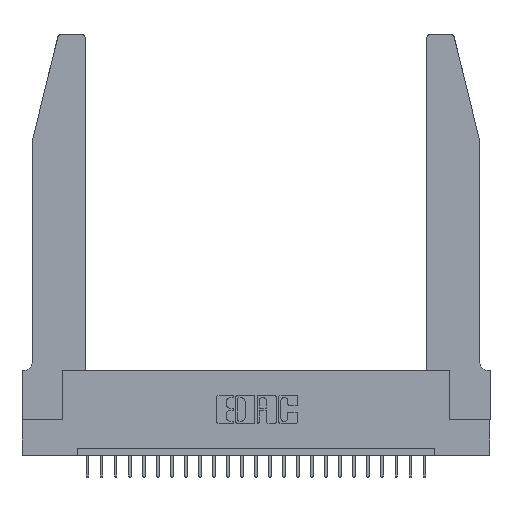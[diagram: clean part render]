
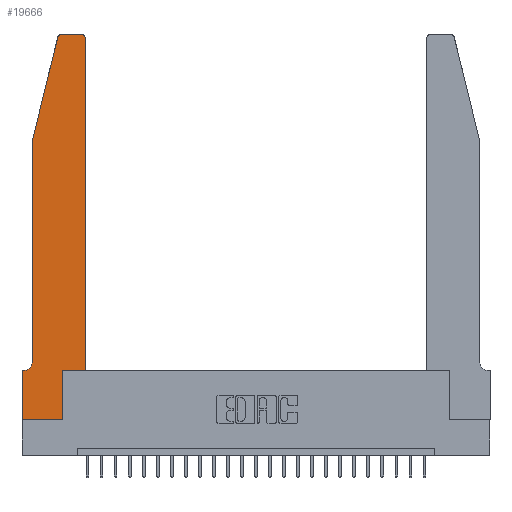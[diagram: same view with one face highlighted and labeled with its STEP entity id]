
A CAD part, top view. The second image highlights one B-rep face of the part: STEP entity #19666.
In plain terms, the highlighted planar face has unit normal (0, 0, 1).
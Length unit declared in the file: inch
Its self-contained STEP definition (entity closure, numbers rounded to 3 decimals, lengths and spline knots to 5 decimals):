
#44 = LINE ( 'NONE', #7718, #8840 ) ;
#342 = EDGE_CURVE ( 'NONE', #24350, #8407, #5939, .T. ) ;
#1142 = VERTEX_POINT ( 'NONE', #2765 ) ;
#1242 = AXIS2_PLACEMENT_3D ( 'NONE', #18867, #20820, #3056 ) ;
#1464 = ORIENTED_EDGE ( 'NONE', *, *, #25532, .T. ) ;
#1854 = DIRECTION ( 'NONE',  ( 0., -1., 0. ) ) ;
#1933 = ORIENTED_EDGE ( 'NONE', *, *, #6863, .T. ) ;
#2113 = AXIS2_PLACEMENT_3D ( 'NONE', #15263, #17402, #19083 ) ;
#2423 = EDGE_CURVE ( 'NONE', #25608, #8100, #19579, .T. ) ;
#2456 = VECTOR ( 'NONE', #14758, 39.37008 ) ;
#2646 = CARTESIAN_POINT ( 'NONE',  ( 0.4205, 2.75, 0.37 ) ) ;
#2706 = CARTESIAN_POINT ( 'NONE',  ( 0.0755, 2., 0.37 ) ) ;
#2765 = CARTESIAN_POINT ( 'NONE',  ( 0., 0., 0.37 ) ) ;
#3056 = DIRECTION ( 'NONE',  ( 1., 0., 0. ) ) ;
#3160 = ORIENTED_EDGE ( 'NONE', *, *, #342, .T. ) ;
#4125 = CARTESIAN_POINT ( 'NONE',  ( 0.4505, 0.35, 0.37 ) ) ;
#4272 = EDGE_CURVE ( 'NONE', #8407, #16023, #17249, .T. ) ;
#4421 = DIRECTION ( 'NONE',  ( 0., 1., 0. ) ) ;
#4674 = CARTESIAN_POINT ( 'NONE',  ( 0.0755, 0.35, 0.37 ) ) ;
#4964 = CARTESIAN_POINT ( 'NONE',  ( 0.0755, 2., 0.37 ) ) ;
#5587 = ORIENTED_EDGE ( 'NONE', *, *, #22084, .T. ) ;
#5939 = LINE ( 'NONE', #22624, #18707 ) ;
#6863 = EDGE_CURVE ( 'NONE', #8203, #24350, #16548, .T. ) ;
#7333 = AXIS2_PLACEMENT_3D ( 'NONE', #18535, #24475, #8673 ) ;
#7586 = AXIS2_PLACEMENT_3D ( 'NONE', #24987, #24915, #12925 ) ;
#7718 = CARTESIAN_POINT ( 'NONE',  ( 0., 0., 0.37 ) ) ;
#7865 = FACE_OUTER_BOUND ( 'NONE', #18715, .T. ) ;
#8100 = VERTEX_POINT ( 'NONE', #4125 ) ;
#8203 = VERTEX_POINT ( 'NONE', #16066 ) ;
#8407 = VERTEX_POINT ( 'NONE', #17975 ) ;
#8673 = DIRECTION ( 'NONE',  ( -1., 0., 0. ) ) ;
#8840 = VECTOR ( 'NONE', #1854, 39.37008 ) ;
#8842 = DIRECTION ( 'NONE',  ( -1., 0., 0. ) ) ;
#8990 = DIRECTION ( 'NONE',  ( 1., 0., 0. ) ) ;
#9147 = EDGE_CURVE ( 'NONE', #17560, #13551, #11936, .T. ) ;
#9151 = DIRECTION ( 'NONE',  ( 1., 0., 0. ) ) ;
#9728 = CARTESIAN_POINT ( 'NONE',  ( 0.0055, 0.35, 0.37 ) ) ;
#9859 = ORIENTED_EDGE ( 'NONE', *, *, #4272, .T. ) ;
#10024 = ORIENTED_EDGE ( 'NONE', *, *, #23371, .T. ) ;
#10175 = VECTOR ( 'NONE', #9151, 39.37008 ) ;
#10719 = VECTOR ( 'NONE', #23475, 39.37008 ) ;
#10767 = CARTESIAN_POINT ( 'NONE',  ( 0.2865, 0.35, 0.37 ) ) ;
#11580 = ORIENTED_EDGE ( 'NONE', *, *, #2423, .T. ) ;
#11936 = LINE ( 'NONE', #21304, #10719 ) ;
#12528 = DIRECTION ( 'NONE',  ( 0., -1., 0. ) ) ;
#12654 = EDGE_CURVE ( 'NONE', #20832, #17560, #21929, .T. ) ;
#12674 = VERTEX_POINT ( 'NONE', #14831 ) ;
#12921 = CARTESIAN_POINT ( 'NONE',  ( 0.4505, 0.35, 0.37 ) ) ;
#12925 = DIRECTION ( 'NONE',  ( 1., 0., 0. ) ) ;
#13551 = VERTEX_POINT ( 'NONE', #17514 ) ;
#14483 = EDGE_CURVE ( 'NONE', #8100, #20832, #14913, .T. ) ;
#14505 = VECTOR ( 'NONE', #8990, 39.37008 ) ;
#14758 = DIRECTION ( 'NONE',  ( 0., 1., 0. ) ) ;
#14831 = CARTESIAN_POINT ( 'NONE',  ( 0.2865, 0., 0.37 ) ) ;
#14913 = LINE ( 'NONE', #12921, #2456 ) ;
#15263 = CARTESIAN_POINT ( 'NONE',  ( 0.284, 2.72, 0.37 ) ) ;
#15326 = EDGE_CURVE ( 'NONE', #16023, #23756, #25230, .T. ) ;
#15534 = VECTOR ( 'NONE', #4421, 39.37008 ) ;
#15767 = ORIENTED_EDGE ( 'NONE', *, *, #12654, .T. ) ;
#16023 = VERTEX_POINT ( 'NONE', #9728 ) ;
#16066 = CARTESIAN_POINT ( 'NONE',  ( 0.25487, 2.72718, 0.37 ) ) ;
#16417 = ORIENTED_EDGE ( 'NONE', *, *, #15326, .T. ) ;
#16506 = CARTESIAN_POINT ( 'NONE',  ( 0.2865, 0.35, 0.37 ) ) ;
#16548 = LINE ( 'NONE', #4964, #19079 ) ;
#17168 = CARTESIAN_POINT ( 'NONE',  ( 0.4505, 0.35, 0.37 ) ) ;
#17249 = CIRCLE ( 'NONE', #7333, 0.07 ) ;
#17402 = DIRECTION ( 'NONE',  ( 0., 0., 1. ) ) ;
#17514 = CARTESIAN_POINT ( 'NONE',  ( 0.284, 2.75, 0.37 ) ) ;
#17560 = VERTEX_POINT ( 'NONE', #2646 ) ;
#17975 = CARTESIAN_POINT ( 'NONE',  ( 0.0755, 0.42, 0.37 ) ) ;
#18037 = VECTOR ( 'NONE', #8842, 39.37008 ) ;
#18535 = CARTESIAN_POINT ( 'NONE',  ( 0.0055, 0.42, 0.37 ) ) ;
#18707 = VECTOR ( 'NONE', #12528, 39.37008 ) ;
#18715 = EDGE_LOOP ( 'NONE', ( #21471, #19552, #1933, #3160, #9859, #16417, #10024, #5587, #1464, #11580, #22810, #15767 ) ) ;
#18867 = CARTESIAN_POINT ( 'NONE',  ( 0.4205, 2.72, 0.37 ) ) ;
#19079 = VECTOR ( 'NONE', #23248, 39.37008 ) ;
#19083 = DIRECTION ( 'NONE',  ( 1., 0., 0. ) ) ;
#19552 = ORIENTED_EDGE ( 'NONE', *, *, #23257, .T. ) ;
#19579 = LINE ( 'NONE', #17168, #14505 ) ;
#19666 = ADVANCED_FACE ( 'NONE', ( #7865 ), #25153, .T. ) ;
#20170 = LINE ( 'NONE', #23131, #10175 ) ;
#20412 = CIRCLE ( 'NONE', #2113, 0.03 ) ;
#20592 = LINE ( 'NONE', #16506, #15534 ) ;
#20743 = CARTESIAN_POINT ( 'NONE',  ( 0., 0.35, 0.37 ) ) ;
#20820 = DIRECTION ( 'NONE',  ( 0., 0., 1. ) ) ;
#20832 = VERTEX_POINT ( 'NONE', #24585 ) ;
#21304 = CARTESIAN_POINT ( 'NONE',  ( 0.2605, 2.75, 0.37 ) ) ;
#21471 = ORIENTED_EDGE ( 'NONE', *, *, #9147, .T. ) ;
#21929 = CIRCLE ( 'NONE', #1242, 0.03 ) ;
#22084 = EDGE_CURVE ( 'NONE', #1142, #12674, #20170, .T. ) ;
#22624 = CARTESIAN_POINT ( 'NONE',  ( 0.0755, 2., 0.37 ) ) ;
#22810 = ORIENTED_EDGE ( 'NONE', *, *, #14483, .T. ) ;
#23131 = CARTESIAN_POINT ( 'NONE',  ( 0., 0., 0.37 ) ) ;
#23248 = DIRECTION ( 'NONE',  ( -0.239, -0.971, 0. ) ) ;
#23257 = EDGE_CURVE ( 'NONE', #13551, #8203, #20412, .T. ) ;
#23371 = EDGE_CURVE ( 'NONE', #23756, #1142, #44, .T. ) ;
#23475 = DIRECTION ( 'NONE',  ( -1., 0., 0. ) ) ;
#23756 = VERTEX_POINT ( 'NONE', #20743 ) ;
#24350 = VERTEX_POINT ( 'NONE', #2706 ) ;
#24475 = DIRECTION ( 'NONE',  ( 0., 0., -1. ) ) ;
#24585 = CARTESIAN_POINT ( 'NONE',  ( 0.4505, 2.72, 0.37 ) ) ;
#24915 = DIRECTION ( 'NONE',  ( 0., 0., 1. ) ) ;
#24987 = CARTESIAN_POINT ( 'NONE',  ( 0., 0.35, 0.37 ) ) ;
#25153 = PLANE ( 'NONE',  #7586 ) ;
#25230 = LINE ( 'NONE', #4674, #18037 ) ;
#25532 = EDGE_CURVE ( 'NONE', #12674, #25608, #20592, .T. ) ;
#25608 = VERTEX_POINT ( 'NONE', #10767 ) ;
